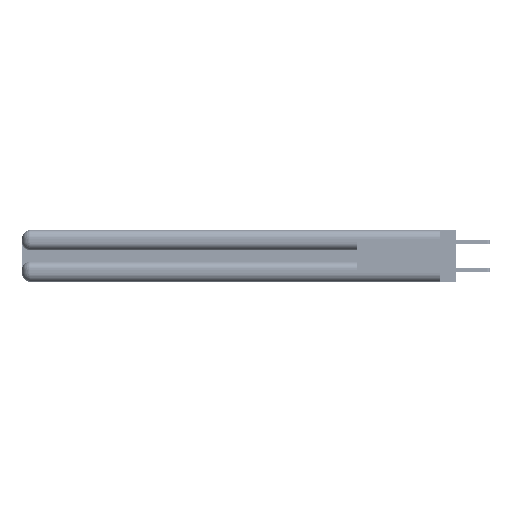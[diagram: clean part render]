
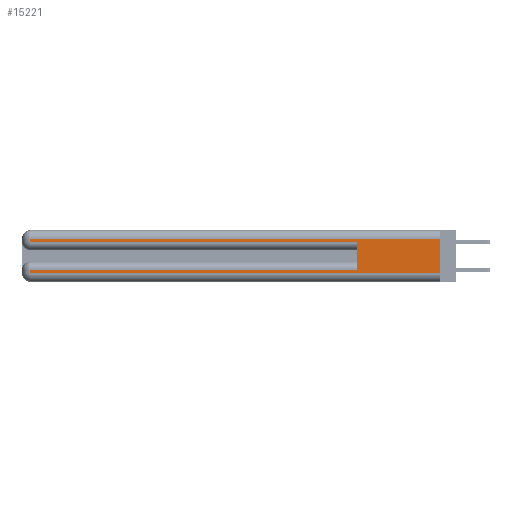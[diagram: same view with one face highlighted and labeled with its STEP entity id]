
A CAD part, left-side view. The second image highlights one B-rep face of the part: STEP entity #15221.
In plain terms, the highlighted planar face has unit normal (-1, 0, 0).
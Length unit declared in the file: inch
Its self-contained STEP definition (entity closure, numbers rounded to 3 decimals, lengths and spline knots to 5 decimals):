
#520 = VECTOR ( 'NONE', #38533, 39.37008 ) ;
#2879 = PLANE ( 'NONE',  #40773 ) ;
#4116 = CARTESIAN_POINT ( 'NONE',  ( 0., 0., 0.31 ) ) ;
#5250 = VERTEX_POINT ( 'NONE', #15176 ) ;
#6734 = CARTESIAN_POINT ( 'NONE',  ( 0., 0., 0.37 ) ) ;
#6871 = VECTOR ( 'NONE', #29779, 39.37008 ) ;
#7359 = VERTEX_POINT ( 'NONE', #15565 ) ;
#7567 = CARTESIAN_POINT ( 'NONE',  ( 0., 0., 0.085 ) ) ;
#8930 = EDGE_CURVE ( 'NONE', #5250, #16492, #41537, .T. ) ;
#9568 = CARTESIAN_POINT ( 'NONE',  ( 0., 2.94, 0.085 ) ) ;
#9846 = ORIENTED_EDGE ( 'NONE', *, *, #24928, .T. ) ;
#10132 = ORIENTED_EDGE ( 'NONE', *, *, #44855, .T. ) ;
#11872 = CARTESIAN_POINT ( 'NONE',  ( 0., 2.94, 0.285 ) ) ;
#12110 = CARTESIAN_POINT ( 'NONE',  ( 0., 0.6, 0.145 ) ) ;
#12420 = FACE_OUTER_BOUND ( 'NONE', #42231, .T. ) ;
#13006 = CARTESIAN_POINT ( 'NONE',  ( 0., 0.6, 0.085 ) ) ;
#14238 = VERTEX_POINT ( 'NONE', #13006 ) ;
#14768 = DIRECTION ( 'NONE',  ( 0., 0., -1. ) ) ;
#15176 = CARTESIAN_POINT ( 'NONE',  ( 0., 0., 0.31 ) ) ;
#15221 = ADVANCED_FACE ( 'NONE', ( #12420 ), #2879, .F. ) ;
#15565 = CARTESIAN_POINT ( 'NONE',  ( 0., 2.94, 0.06 ) ) ;
#16208 = EDGE_CURVE ( 'NONE', #49191, #28998, #48515, .T. ) ;
#16492 = VERTEX_POINT ( 'NONE', #47355 ) ;
#17111 = CARTESIAN_POINT ( 'NONE',  ( 0., 2.94, 0.37 ) ) ;
#18394 = ORIENTED_EDGE ( 'NONE', *, *, #26804, .T. ) ;
#18935 = VERTEX_POINT ( 'NONE', #25167 ) ;
#18990 = ORIENTED_EDGE ( 'NONE', *, *, #8930, .F. ) ;
#19254 = VECTOR ( 'NONE', #41797, 39.37008 ) ;
#19331 = DIRECTION ( 'NONE',  ( 0., -1., 0. ) ) ;
#19546 = LINE ( 'NONE', #17111, #30860 ) ;
#21051 = DIRECTION ( 'NONE',  ( 0., 0., -1. ) ) ;
#21764 = VECTOR ( 'NONE', #19331, 39.37008 ) ;
#23455 = EDGE_CURVE ( 'NONE', #14238, #29407, #29371, .T. ) ;
#24928 = EDGE_CURVE ( 'NONE', #29407, #7359, #19546, .T. ) ;
#25167 = CARTESIAN_POINT ( 'NONE',  ( 0., 2.94, 0.31 ) ) ;
#26371 = ORIENTED_EDGE ( 'NONE', *, *, #27394, .F. ) ;
#26804 = EDGE_CURVE ( 'NONE', #7359, #16492, #29478, .T. ) ;
#27394 = EDGE_CURVE ( 'NONE', #14238, #28998, #31762, .T. ) ;
#28371 = CARTESIAN_POINT ( 'NONE',  ( 0., 0.6, 0.285 ) ) ;
#28898 = ORIENTED_EDGE ( 'NONE', *, *, #42049, .T. ) ;
#28998 = VERTEX_POINT ( 'NONE', #28371 ) ;
#29371 = LINE ( 'NONE', #7567, #19254 ) ;
#29407 = VERTEX_POINT ( 'NONE', #9568 ) ;
#29478 = LINE ( 'NONE', #40913, #6871 ) ;
#29779 = DIRECTION ( 'NONE',  ( 0., -1., 0. ) ) ;
#30860 = VECTOR ( 'NONE', #21051, 39.37008 ) ;
#31762 = LINE ( 'NONE', #12110, #44222 ) ;
#32753 = ORIENTED_EDGE ( 'NONE', *, *, #23455, .T. ) ;
#33311 = DIRECTION ( 'NONE',  ( 1., 0., 0. ) ) ;
#34817 = DIRECTION ( 'NONE',  ( 0., 0., -1. ) ) ;
#36824 = VECTOR ( 'NONE', #34817, 39.37008 ) ;
#37095 = LINE ( 'NONE', #4116, #520 ) ;
#37505 = CARTESIAN_POINT ( 'NONE',  ( 0., 2.94, 0.37 ) ) ;
#38533 = DIRECTION ( 'NONE',  ( 0., 1., 0. ) ) ;
#38681 = DIRECTION ( 'NONE',  ( 0., 0., 1. ) ) ;
#38927 = CARTESIAN_POINT ( 'NONE',  ( 0., 0., 0.285 ) ) ;
#40773 = AXIS2_PLACEMENT_3D ( 'NONE', #6734, #33311, #47773 ) ;
#40913 = CARTESIAN_POINT ( 'NONE',  ( 0., 0., 0.06 ) ) ;
#41537 = LINE ( 'NONE', #46440, #36824 ) ;
#41797 = DIRECTION ( 'NONE',  ( 0., 1., 0. ) ) ;
#41895 = ORIENTED_EDGE ( 'NONE', *, *, #16208, .T. ) ;
#42049 = EDGE_CURVE ( 'NONE', #5250, #18935, #37095, .T. ) ;
#42231 = EDGE_LOOP ( 'NONE', ( #18990, #28898, #10132, #41895, #26371, #32753, #9846, #18394 ) ) ;
#42969 = LINE ( 'NONE', #37505, #44153 ) ;
#44153 = VECTOR ( 'NONE', #14768, 39.37008 ) ;
#44222 = VECTOR ( 'NONE', #38681, 39.37008 ) ;
#44855 = EDGE_CURVE ( 'NONE', #18935, #49191, #42969, .T. ) ;
#46440 = CARTESIAN_POINT ( 'NONE',  ( 0., 0., 0.37 ) ) ;
#47355 = CARTESIAN_POINT ( 'NONE',  ( 0., 0., 0.06 ) ) ;
#47773 = DIRECTION ( 'NONE',  ( 0., 0., -1. ) ) ;
#48515 = LINE ( 'NONE', #38927, #21764 ) ;
#49191 = VERTEX_POINT ( 'NONE', #11872 ) ;
